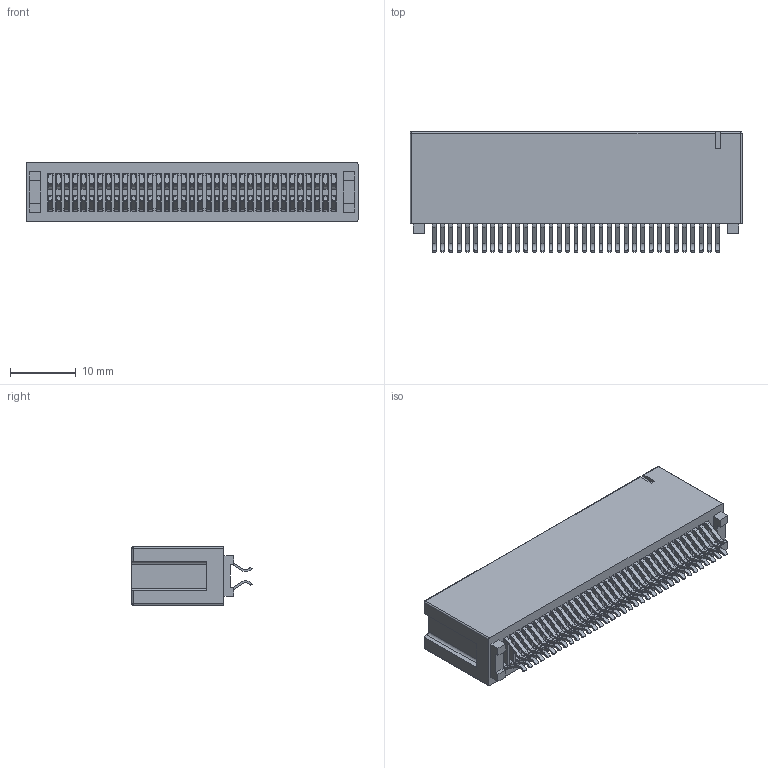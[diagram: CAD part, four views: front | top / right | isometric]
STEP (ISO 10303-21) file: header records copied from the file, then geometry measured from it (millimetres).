
FILE_DESCRIPTION (( 'STEP AP203' ), '1' );
FILE_NAME ('302-070-656-201.STEP', '2024-04-06T05:35:55', ( '' ), ( '' ), 'SwSTEP 2.0', 'SolidWorks 2023', '' );
FILE_SCHEMA (( 'CONFIG_CONTROL_DESIGN' ));
Length unit declared in the file: millimetre
Products named in the file (3): 302-070-656-201; Contact_302-290-X56; HSG_Vertical HSG
Assembly tree (71 placements, depth 2):
  302-070-656-201
    HSG_Vertical HSG
    Contact_302-290-X56  x70
Bounding box: 50.55 x 18.3 x 8.88 mm (x, y, z)
Volume: 3941.3 mm3; surface area: 10855 mm2
Topology: 71 solids, 71 shells, 3391 faces, 10108 edges, 6684 vertices
Faces by surface type: plane 2254, cylinder 1133, sphere 4
Entity records: 27645 total; most frequent: ORIENTED_EDGE 4752, CARTESIAN_POINT 4679, DIRECTION 3836, EDGE_CURVE 2376, VECTOR 2318, LINE 2318, VERTEX_POINT 1578, AXIS2_PLACEMENT_3D 759
